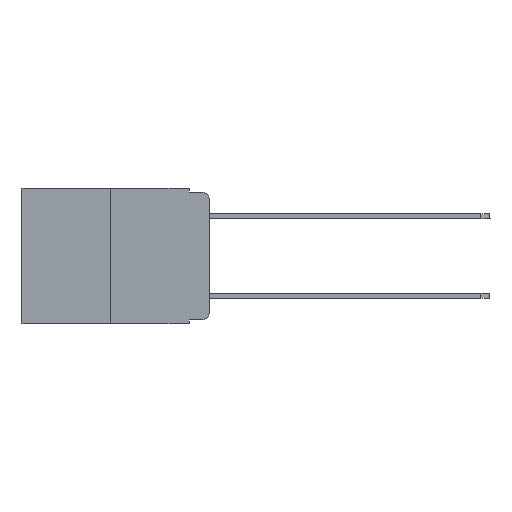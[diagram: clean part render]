
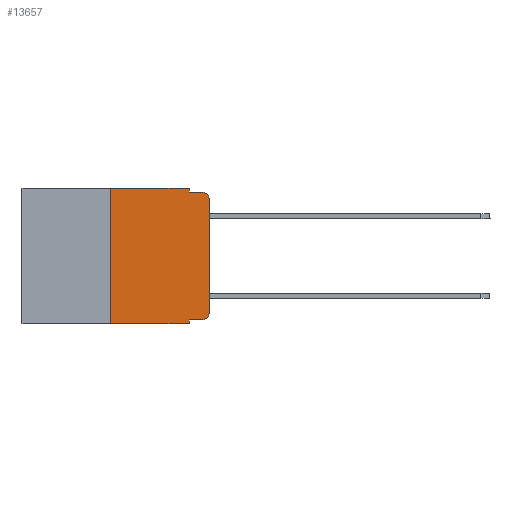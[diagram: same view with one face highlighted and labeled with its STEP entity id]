
A CAD part, left-side view. The second image highlights one B-rep face of the part: STEP entity #13657.
In plain terms, the highlighted planar face has unit normal (-1, 0, 0).
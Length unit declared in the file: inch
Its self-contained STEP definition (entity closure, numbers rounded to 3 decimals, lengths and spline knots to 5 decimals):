
#80 = ORIENTED_EDGE ( 'NONE', *, *, #3385, .T. ) ;
#237 = DIRECTION ( 'NONE',  ( 0., -1., 0. ) ) ;
#437 = CARTESIAN_POINT ( 'NONE',  ( 0., 0., -0.313 ) ) ;
#1216 = LINE ( 'NONE', #1914, #13808 ) ;
#1271 = AXIS2_PLACEMENT_3D ( 'NONE', #11228, #5282, #19008 ) ;
#1586 = LINE ( 'NONE', #10722, #15397 ) ;
#1756 = VERTEX_POINT ( 'NONE', #18141 ) ;
#1863 = LINE ( 'NONE', #7238, #14951 ) ;
#1914 = CARTESIAN_POINT ( 'NONE',  ( 0., 0.473, 0. ) ) ;
#2041 = ORIENTED_EDGE ( 'NONE', *, *, #15891, .T. ) ;
#2228 = DIRECTION ( 'NONE',  ( 0., 0., -1. ) ) ;
#2559 = AXIS2_PLACEMENT_3D ( 'NONE', #16239, #11378, #2228 ) ;
#2815 = EDGE_CURVE ( 'NONE', #9453, #11967, #16210, .T. ) ;
#3208 = EDGE_LOOP ( 'NONE', ( #17509, #80, #17521, #15584, #11977, #12713, #19713, #13972, #2041, #4514 ) ) ;
#3385 = EDGE_CURVE ( 'NONE', #13793, #19753, #6414, .T. ) ;
#3543 = CARTESIAN_POINT ( 'NONE',  ( 0., 0.473, 0. ) ) ;
#4205 = CIRCLE ( 'NONE', #1271, 0.02 ) ;
#4514 = ORIENTED_EDGE ( 'NONE', *, *, #5502, .T. ) ;
#4808 = VERTEX_POINT ( 'NONE', #437 ) ;
#5013 = LINE ( 'NONE', #6110, #10339 ) ;
#5282 = DIRECTION ( 'NONE',  ( -1., 0., 0. ) ) ;
#5502 = EDGE_CURVE ( 'NONE', #19557, #4808, #4205, .T. ) ;
#5596 = CARTESIAN_POINT ( 'NONE',  ( 0., 0.02, -0.333 ) ) ;
#5665 = CARTESIAN_POINT ( 'NONE',  ( 0., 0., -0.03 ) ) ;
#5761 = CARTESIAN_POINT ( 'NONE',  ( 0., 0.051, -0.343 ) ) ;
#5847 = CARTESIAN_POINT ( 'NONE',  ( 0., 0.051, -0.01 ) ) ;
#5958 = VECTOR ( 'NONE', #12226, 39.37008 ) ;
#6110 = CARTESIAN_POINT ( 'NONE',  ( 0., 0.051, 0. ) ) ;
#6414 = CIRCLE ( 'NONE', #2559, 0.02 ) ;
#6917 = VERTEX_POINT ( 'NONE', #15624 ) ;
#7238 = CARTESIAN_POINT ( 'NONE',  ( 0., 0.25, 0. ) ) ;
#7836 = CARTESIAN_POINT ( 'NONE',  ( 0., 0.473, -0.343 ) ) ;
#8047 = EDGE_CURVE ( 'NONE', #1756, #6917, #1863, .T. ) ;
#8210 = DIRECTION ( 'NONE',  ( 0., 0., -1. ) ) ;
#9217 = LINE ( 'NONE', #16722, #17262 ) ;
#9453 = VERTEX_POINT ( 'NONE', #18295 ) ;
#9466 = VERTEX_POINT ( 'NONE', #20053 ) ;
#9888 = DIRECTION ( 'NONE',  ( 1., 0., 0. ) ) ;
#10339 = VECTOR ( 'NONE', #15447, 39.37008 ) ;
#10545 = EDGE_CURVE ( 'NONE', #6917, #9453, #1216, .T. ) ;
#10722 = CARTESIAN_POINT ( 'NONE',  ( 0., 0., 0. ) ) ;
#10758 = VERTEX_POINT ( 'NONE', #5761 ) ;
#11206 = CARTESIAN_POINT ( 'NONE',  ( 0., 0.051, 0. ) ) ;
#11228 = CARTESIAN_POINT ( 'NONE',  ( 0., 0.02, -0.313 ) ) ;
#11378 = DIRECTION ( 'NONE',  ( -1., 0., 0. ) ) ;
#11814 = VECTOR ( 'NONE', #8210, 39.37008 ) ;
#11872 = DIRECTION ( 'NONE',  ( 0., 0., 1. ) ) ;
#11967 = VERTEX_POINT ( 'NONE', #5847 ) ;
#11977 = ORIENTED_EDGE ( 'NONE', *, *, #10545, .F. ) ;
#12070 = DIRECTION ( 'NONE',  ( 0., -1., 0. ) ) ;
#12118 = EDGE_CURVE ( 'NONE', #9466, #10758, #5013, .T. ) ;
#12226 = DIRECTION ( 'NONE',  ( 0., -1., 0. ) ) ;
#12701 = EDGE_CURVE ( 'NONE', #11967, #19753, #9217, .T. ) ;
#12713 = ORIENTED_EDGE ( 'NONE', *, *, #8047, .F. ) ;
#12802 = EDGE_CURVE ( 'NONE', #1756, #10758, #14090, .T. ) ;
#12806 = PLANE ( 'NONE',  #18464 ) ;
#13520 = LINE ( 'NONE', #15312, #5958 ) ;
#13587 = FACE_OUTER_BOUND ( 'NONE', #3208, .T. ) ;
#13657 = ADVANCED_FACE ( 'NONE', ( #13587 ), #12806, .F. ) ;
#13793 = VERTEX_POINT ( 'NONE', #5665 ) ;
#13808 = VECTOR ( 'NONE', #15848, 39.37008 ) ;
#13933 = CARTESIAN_POINT ( 'NONE',  ( 0., 0.02, -0.01 ) ) ;
#13972 = ORIENTED_EDGE ( 'NONE', *, *, #12118, .F. ) ;
#14090 = LINE ( 'NONE', #7836, #15561 ) ;
#14380 = DIRECTION ( 'NONE',  ( 0., 0., -1. ) ) ;
#14951 = VECTOR ( 'NONE', #11872, 39.37008 ) ;
#15312 = CARTESIAN_POINT ( 'NONE',  ( 0., 0.051, -0.333 ) ) ;
#15397 = VECTOR ( 'NONE', #19983, 39.37008 ) ;
#15447 = DIRECTION ( 'NONE',  ( 0., 0., -1. ) ) ;
#15561 = VECTOR ( 'NONE', #237, 39.37008 ) ;
#15584 = ORIENTED_EDGE ( 'NONE', *, *, #2815, .F. ) ;
#15624 = CARTESIAN_POINT ( 'NONE',  ( 0., 0.25, 0. ) ) ;
#15848 = DIRECTION ( 'NONE',  ( 0., -1., 0. ) ) ;
#15891 = EDGE_CURVE ( 'NONE', #9466, #19557, #13520, .T. ) ;
#16210 = LINE ( 'NONE', #11206, #11814 ) ;
#16239 = CARTESIAN_POINT ( 'NONE',  ( 0., 0.02, -0.03 ) ) ;
#16722 = CARTESIAN_POINT ( 'NONE',  ( 0., 0.051, -0.01 ) ) ;
#17262 = VECTOR ( 'NONE', #12070, 39.37008 ) ;
#17397 = EDGE_CURVE ( 'NONE', #4808, #13793, #1586, .T. ) ;
#17509 = ORIENTED_EDGE ( 'NONE', *, *, #17397, .T. ) ;
#17521 = ORIENTED_EDGE ( 'NONE', *, *, #12701, .F. ) ;
#18141 = CARTESIAN_POINT ( 'NONE',  ( 0., 0.25, -0.343 ) ) ;
#18295 = CARTESIAN_POINT ( 'NONE',  ( 0., 0.051, 0. ) ) ;
#18464 = AXIS2_PLACEMENT_3D ( 'NONE', #3543, #9888, #14380 ) ;
#19008 = DIRECTION ( 'NONE',  ( 0., 0., -1. ) ) ;
#19557 = VERTEX_POINT ( 'NONE', #5596 ) ;
#19713 = ORIENTED_EDGE ( 'NONE', *, *, #12802, .T. ) ;
#19753 = VERTEX_POINT ( 'NONE', #13933 ) ;
#19983 = DIRECTION ( 'NONE',  ( 0., 0., 1. ) ) ;
#20053 = CARTESIAN_POINT ( 'NONE',  ( 0., 0.051, -0.333 ) ) ;
